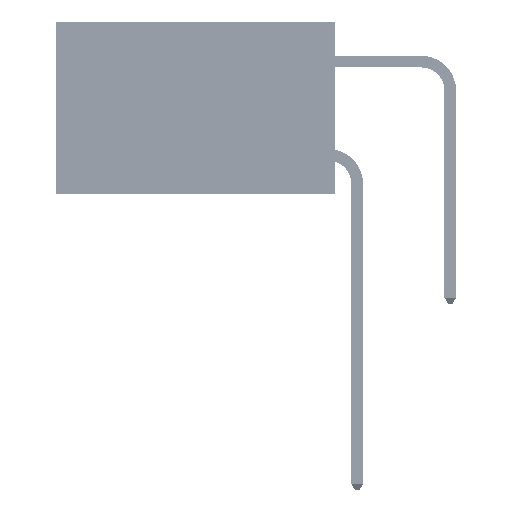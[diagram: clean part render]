
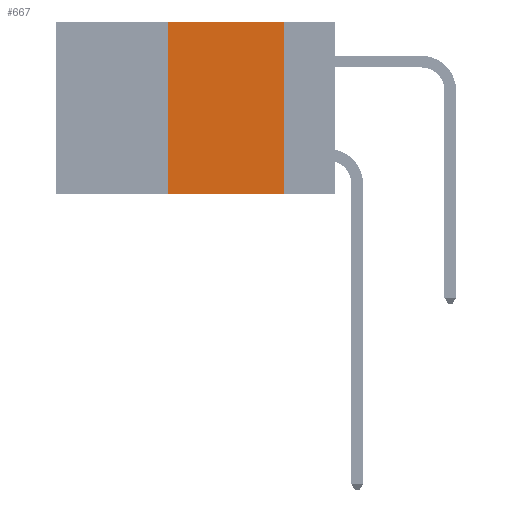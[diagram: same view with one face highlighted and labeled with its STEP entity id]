
A CAD part, left-side view. The second image highlights one B-rep face of the part: STEP entity #667.
In plain terms, the highlighted planar face has unit normal (-1, 0, 0).
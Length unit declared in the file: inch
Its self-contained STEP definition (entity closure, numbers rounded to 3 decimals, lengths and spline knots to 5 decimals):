
#155 = VECTOR ( 'NONE', #32421, 39.37008 ) ;
#458 = CARTESIAN_POINT ( 'NONE',  ( 0., 0.36, -0.37 ) ) ;
#667 = ADVANCED_FACE ( 'NONE', ( #28705 ), #29275, .F. ) ;
#1618 = CARTESIAN_POINT ( 'NONE',  ( 0., 0.11, -0.37 ) ) ;
#2173 = EDGE_CURVE ( 'NONE', #33415, #24379, #18977, .T. ) ;
#3002 = VERTEX_POINT ( 'NONE', #1618 ) ;
#3106 = ORIENTED_EDGE ( 'NONE', *, *, #2173, .F. ) ;
#3817 = EDGE_CURVE ( 'NONE', #33415, #3002, #44391, .T. ) ;
#4155 = CARTESIAN_POINT ( 'NONE',  ( 0., 0.6, 0. ) ) ;
#8531 = VECTOR ( 'NONE', #39884, 39.37008 ) ;
#10830 = DIRECTION ( 'NONE',  ( 1., 0., 0. ) ) ;
#10836 = VERTEX_POINT ( 'NONE', #39093 ) ;
#11231 = AXIS2_PLACEMENT_3D ( 'NONE', #4155, #10830, #39922 ) ;
#11357 = VECTOR ( 'NONE', #33591, 39.37008 ) ;
#12451 = VECTOR ( 'NONE', #42834, 39.37008 ) ;
#15068 = CARTESIAN_POINT ( 'NONE',  ( 0., 0.36, 0. ) ) ;
#18143 = LINE ( 'NONE', #35817, #12451 ) ;
#18977 = LINE ( 'NONE', #15068, #155 ) ;
#22160 = EDGE_LOOP ( 'NONE', ( #27120, #27025, #3106, #35192 ) ) ;
#24379 = VERTEX_POINT ( 'NONE', #29430 ) ;
#27025 = ORIENTED_EDGE ( 'NONE', *, *, #34512, .F. ) ;
#27120 = ORIENTED_EDGE ( 'NONE', *, *, #42679, .F. ) ;
#28705 = FACE_OUTER_BOUND ( 'NONE', #22160, .T. ) ;
#29275 = PLANE ( 'NONE',  #11231 ) ;
#29430 = CARTESIAN_POINT ( 'NONE',  ( 0., 0.36, 0. ) ) ;
#32421 = DIRECTION ( 'NONE',  ( 0., 0., 1. ) ) ;
#32957 = LINE ( 'NONE', #47042, #8531 ) ;
#33415 = VERTEX_POINT ( 'NONE', #458 ) ;
#33591 = DIRECTION ( 'NONE',  ( 0., -1., 0. ) ) ;
#34512 = EDGE_CURVE ( 'NONE', #24379, #10836, #18143, .T. ) ;
#35192 = ORIENTED_EDGE ( 'NONE', *, *, #3817, .T. ) ;
#35817 = CARTESIAN_POINT ( 'NONE',  ( 0., 0.6, 0. ) ) ;
#39093 = CARTESIAN_POINT ( 'NONE',  ( 0., 0.11, 0. ) ) ;
#39884 = DIRECTION ( 'NONE',  ( 0., 0., -1. ) ) ;
#39922 = DIRECTION ( 'NONE',  ( 0., 0., -1. ) ) ;
#41232 = CARTESIAN_POINT ( 'NONE',  ( 0., 0.6, -0.37 ) ) ;
#42679 = EDGE_CURVE ( 'NONE', #10836, #3002, #32957, .T. ) ;
#42834 = DIRECTION ( 'NONE',  ( 0., -1., 0. ) ) ;
#44391 = LINE ( 'NONE', #41232, #11357 ) ;
#47042 = CARTESIAN_POINT ( 'NONE',  ( 0., 0.11, 0. ) ) ;
